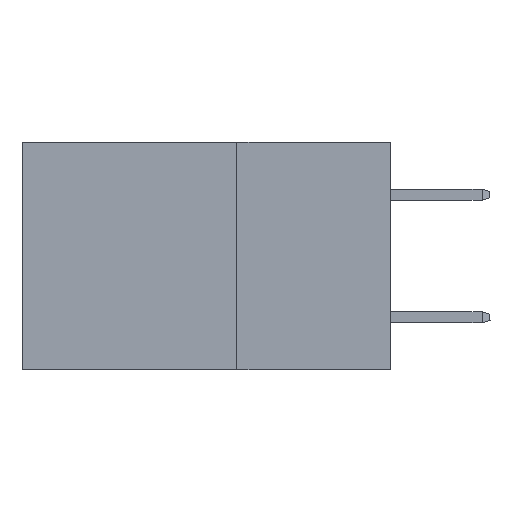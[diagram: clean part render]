
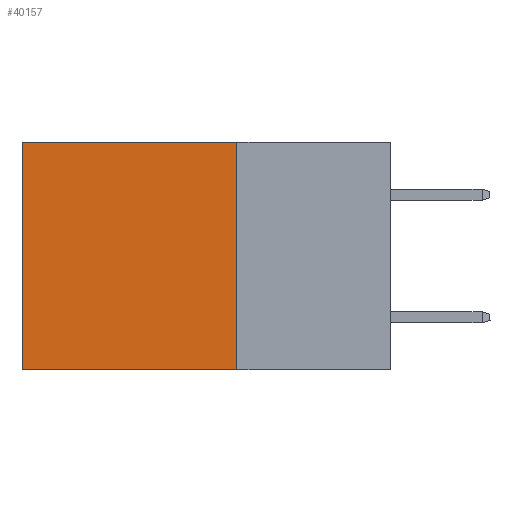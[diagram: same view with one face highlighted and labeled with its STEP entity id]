
A CAD part, left-side view. The second image highlights one B-rep face of the part: STEP entity #40157.
In plain terms, the highlighted planar face has unit normal (-1, 0, 0).
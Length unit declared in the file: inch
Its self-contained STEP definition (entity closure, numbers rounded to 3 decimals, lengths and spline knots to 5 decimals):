
#996 = CARTESIAN_POINT ( 'NONE',  ( 0.2875, 0.25, 0. ) ) ;
#1839 = PLANE ( 'NONE',  #5532 ) ;
#3537 = VECTOR ( 'NONE', #9394, 39.37008 ) ;
#3599 = LINE ( 'NONE', #10569, #43336 ) ;
#5532 = AXIS2_PLACEMENT_3D ( 'NONE', #11770, #36119, #37658 ) ;
#5999 = CARTESIAN_POINT ( 'NONE',  ( 0.2875, 0.25, -0.37 ) ) ;
#7180 = EDGE_LOOP ( 'NONE', ( #26233, #22326, #11180, #21292 ) ) ;
#7784 = VERTEX_POINT ( 'NONE', #41749 ) ;
#9394 = DIRECTION ( 'NONE',  ( 0., 1., 0. ) ) ;
#10118 = LINE ( 'NONE', #23885, #32321 ) ;
#10569 = CARTESIAN_POINT ( 'NONE',  ( 0.2875, 0.6, 0. ) ) ;
#11180 = ORIENTED_EDGE ( 'NONE', *, *, #13293, .F. ) ;
#11770 = CARTESIAN_POINT ( 'NONE',  ( 0.2875, 0.25, 0. ) ) ;
#13293 = EDGE_CURVE ( 'NONE', #21063, #15595, #27064, .T. ) ;
#13508 = VECTOR ( 'NONE', #34276, 39.37008 ) ;
#13755 = DIRECTION ( 'NONE',  ( 0., 0., -1. ) ) ;
#15595 = VERTEX_POINT ( 'NONE', #5999 ) ;
#17346 = EDGE_CURVE ( 'NONE', #7784, #18474, #3599, .T. ) ;
#18474 = VERTEX_POINT ( 'NONE', #26617 ) ;
#20512 = DIRECTION ( 'NONE',  ( 0., 1., 0. ) ) ;
#21063 = VERTEX_POINT ( 'NONE', #996 ) ;
#21292 = ORIENTED_EDGE ( 'NONE', *, *, #35254, .T. ) ;
#21945 = FACE_OUTER_BOUND ( 'NONE', #7180, .T. ) ;
#22326 = ORIENTED_EDGE ( 'NONE', *, *, #30102, .F. ) ;
#23885 = CARTESIAN_POINT ( 'NONE',  ( 0.2875, 0.25, 0. ) ) ;
#26233 = ORIENTED_EDGE ( 'NONE', *, *, #17346, .T. ) ;
#26617 = CARTESIAN_POINT ( 'NONE',  ( 0.2875, 0.6, -0.37 ) ) ;
#26844 = CARTESIAN_POINT ( 'NONE',  ( 0.2875, 0.25, 0. ) ) ;
#27064 = LINE ( 'NONE', #26844, #13508 ) ;
#29935 = LINE ( 'NONE', #40262, #3537 ) ;
#30102 = EDGE_CURVE ( 'NONE', #15595, #18474, #29935, .T. ) ;
#32321 = VECTOR ( 'NONE', #20512, 39.37008 ) ;
#34276 = DIRECTION ( 'NONE',  ( 0., 0., -1. ) ) ;
#35254 = EDGE_CURVE ( 'NONE', #21063, #7784, #10118, .T. ) ;
#36119 = DIRECTION ( 'NONE',  ( 1., 0., 0. ) ) ;
#37658 = DIRECTION ( 'NONE',  ( 0., 0., -1. ) ) ;
#40157 = ADVANCED_FACE ( 'NONE', ( #21945 ), #1839, .F. ) ;
#40262 = CARTESIAN_POINT ( 'NONE',  ( 0.2875, 0.25, -0.37 ) ) ;
#41749 = CARTESIAN_POINT ( 'NONE',  ( 0.2875, 0.6, 0. ) ) ;
#43336 = VECTOR ( 'NONE', #13755, 39.37008 ) ;
